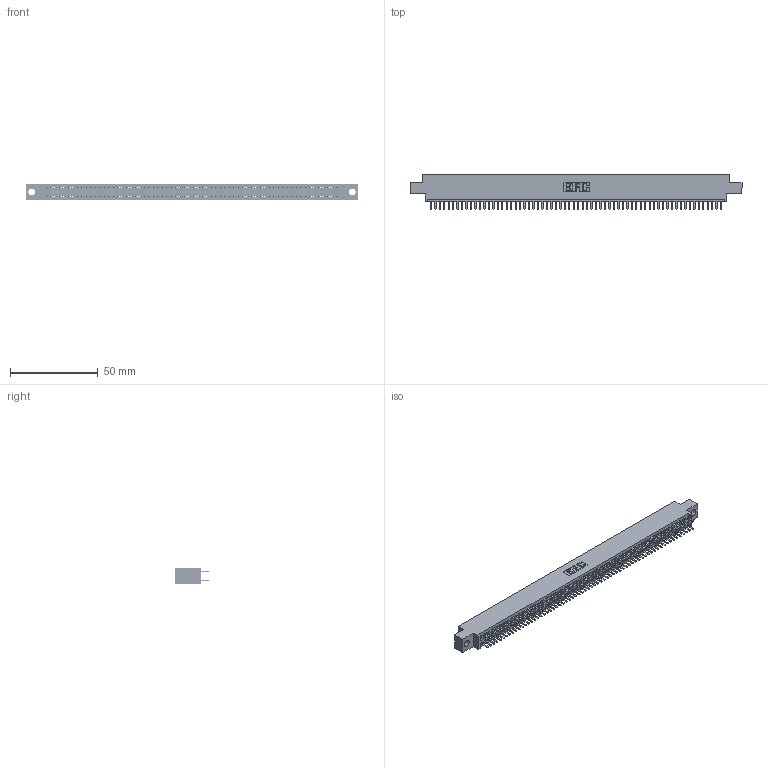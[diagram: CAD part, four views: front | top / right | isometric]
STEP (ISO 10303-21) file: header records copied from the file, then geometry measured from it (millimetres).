
FILE_DESCRIPTION (( 'STEP AP203' ), '1' );
FILE_NAME ('395-132-520-804.STEP', '2021-06-18T00:51:35', ( '' ), ( '' ), 'SwSTEP 2.0', 'SolidWorks 2020', '' );
FILE_SCHEMA (( 'CONFIG_CONTROL_DESIGN' ));
Length unit declared in the file: inch
Products named in the file (3): 345 Part_0.170 Offset - 0.156 Dia-TI; 395-132-520-804; 345-292-001_345-293-120
Assembly tree (133 placements, depth 2):
  395-132-520-804
    345 Part_0.170 Offset - 0.156 Dia-TI
    345-292-001_345-293-120  x132
Bounding box: 188.85 x 19.68 x 9.4 mm (x, y, z)
Volume: 18290.4 mm3; surface area: 27372.8 mm2
Topology: 133 solids, 133 shells, 7272 faces, 21113 edges, 13722 vertices
Faces by surface type: plane 4718, cylinder 2554
Entity records: 49219 total; most frequent: CARTESIAN_POINT 8246, ORIENTED_EDGE 8166, DIRECTION 7227, EDGE_CURVE 4083, LINE 3683, VECTOR 3683, VERTEX_POINT 2718, AXIS2_PLACEMENT_3D 1772
